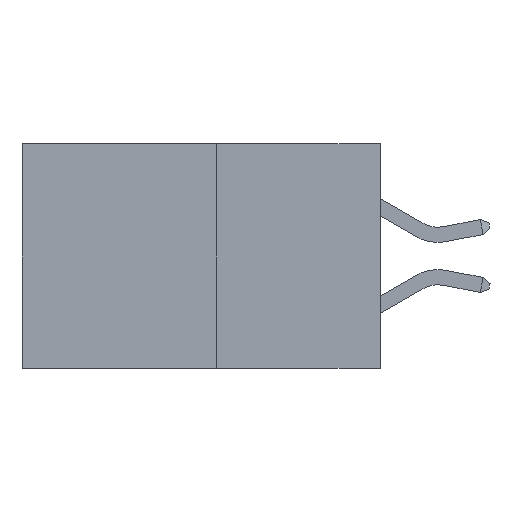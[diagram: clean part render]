
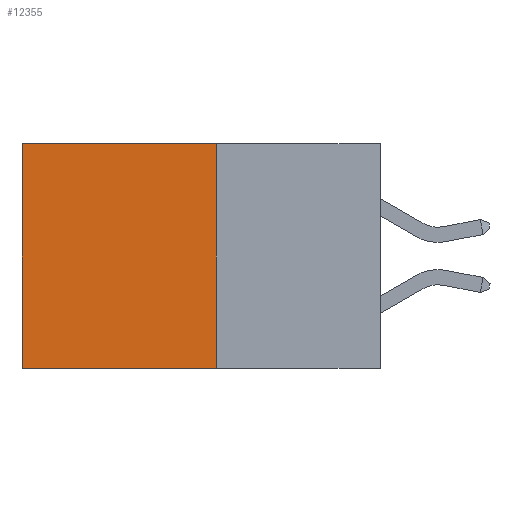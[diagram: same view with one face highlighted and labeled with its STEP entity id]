
A CAD part, left-side view. The second image highlights one B-rep face of the part: STEP entity #12355.
In plain terms, the highlighted planar face has unit normal (-1, 0, 0).
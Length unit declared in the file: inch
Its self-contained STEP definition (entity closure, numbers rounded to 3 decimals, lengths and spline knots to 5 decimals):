
#651 = CARTESIAN_POINT ( 'NONE',  ( 0.277, 0.27, -0.37 ) ) ;
#1213 = ORIENTED_EDGE ( 'NONE', *, *, #23742, .F. ) ;
#2063 = CARTESIAN_POINT ( 'NONE',  ( 0.277, 0.59, -0.37 ) ) ;
#2253 = CARTESIAN_POINT ( 'NONE',  ( 0.277, 0.27, -0.37 ) ) ;
#2510 = DIRECTION ( 'NONE',  ( 0., 1., 0. ) ) ;
#2977 = CARTESIAN_POINT ( 'NONE',  ( 0.277, 0.59, -0.37 ) ) ;
#3360 = DIRECTION ( 'NONE',  ( 0., 1., 0. ) ) ;
#3794 = LINE ( 'NONE', #651, #30490 ) ;
#5268 = VERTEX_POINT ( 'NONE', #32606 ) ;
#5300 = LINE ( 'NONE', #18478, #33636 ) ;
#5486 = LINE ( 'NONE', #2977, #32165 ) ;
#8857 = DIRECTION ( 'NONE',  ( 0., 0., -1. ) ) ;
#10321 = PLANE ( 'NONE',  #22491 ) ;
#11547 = VERTEX_POINT ( 'NONE', #2063 ) ;
#11556 = CARTESIAN_POINT ( 'NONE',  ( 0.277, 0.27, -0.37 ) ) ;
#11814 = EDGE_CURVE ( 'NONE', #16792, #11547, #5486, .T. ) ;
#12355 = ADVANCED_FACE ( 'NONE', ( #16288 ), #10321, .F. ) ;
#13804 = EDGE_CURVE ( 'NONE', #5268, #16792, #5300, .T. ) ;
#15477 = LINE ( 'NONE', #11556, #28822 ) ;
#15675 = DIRECTION ( 'NONE',  ( 1., 0., 0. ) ) ;
#16288 = FACE_OUTER_BOUND ( 'NONE', #34455, .T. ) ;
#16524 = CARTESIAN_POINT ( 'NONE',  ( 0.277, 0.27, -0.37 ) ) ;
#16792 = VERTEX_POINT ( 'NONE', #21115 ) ;
#18478 = CARTESIAN_POINT ( 'NONE',  ( 0.277, 0.27, 0. ) ) ;
#21115 = CARTESIAN_POINT ( 'NONE',  ( 0.277, 0.59, 0. ) ) ;
#21640 = DIRECTION ( 'NONE',  ( 0., 0., -1. ) ) ;
#22202 = ORIENTED_EDGE ( 'NONE', *, *, #23703, .F. ) ;
#22345 = ORIENTED_EDGE ( 'NONE', *, *, #13804, .T. ) ;
#22491 = AXIS2_PLACEMENT_3D ( 'NONE', #2253, #15675, #34254 ) ;
#23703 = EDGE_CURVE ( 'NONE', #29296, #11547, #3794, .T. ) ;
#23742 = EDGE_CURVE ( 'NONE', #5268, #29296, #15477, .T. ) ;
#28822 = VECTOR ( 'NONE', #8857, 39.37008 ) ;
#29296 = VERTEX_POINT ( 'NONE', #16524 ) ;
#30490 = VECTOR ( 'NONE', #3360, 39.37008 ) ;
#30512 = ORIENTED_EDGE ( 'NONE', *, *, #11814, .T. ) ;
#32165 = VECTOR ( 'NONE', #21640, 39.37008 ) ;
#32606 = CARTESIAN_POINT ( 'NONE',  ( 0.277, 0.27, 0. ) ) ;
#33636 = VECTOR ( 'NONE', #2510, 39.37008 ) ;
#34254 = DIRECTION ( 'NONE',  ( 0., 0., -1. ) ) ;
#34455 = EDGE_LOOP ( 'NONE', ( #30512, #22202, #1213, #22345 ) ) ;
